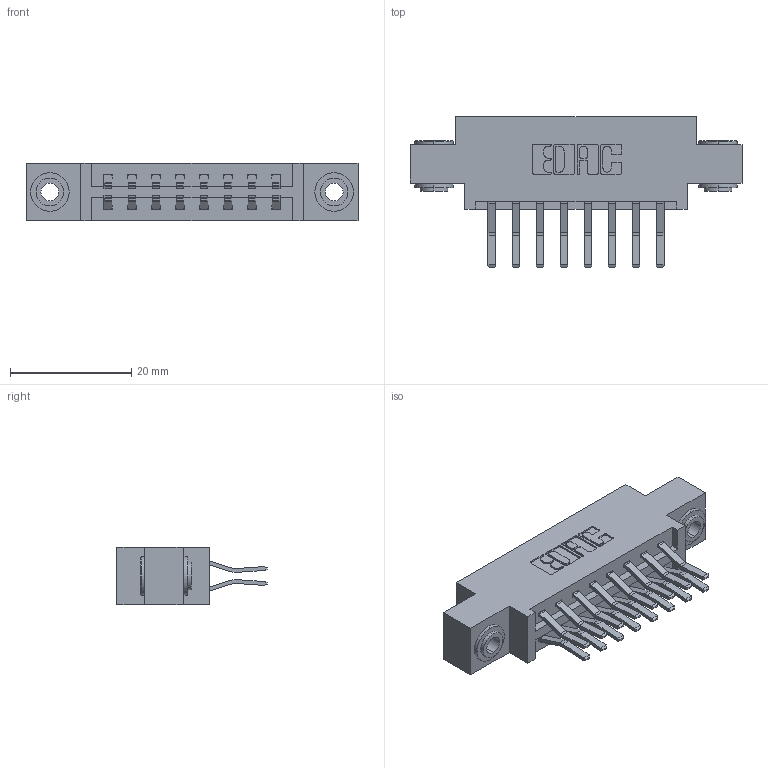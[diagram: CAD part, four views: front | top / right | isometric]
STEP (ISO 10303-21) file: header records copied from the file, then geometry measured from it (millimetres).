
FILE_DESCRIPTION (( 'STEP AP203' ), '1' );
FILE_NAME ('337-016-560-803.STEP', '2019-10-10T18:24:27', ( '' ), ( '' ), 'SwSTEP 2.0', 'SolidWorks 2016', '' );
FILE_SCHEMA (( 'CONFIG_CONTROL_DESIGN' ));
Length unit declared in the file: inch
Products named in the file (4): 345-250-002_345-250-002-102; 345-292-001_560 Tail; 337 Part_0.170 Offset - 0.156 Dia-TH; 337-016-560-803
Assembly tree (19 placements, depth 2):
  337-016-560-803
    337 Part_0.170 Offset - 0.156 Dia-TH
    345-292-001_560 Tail  x16
    345-250-002_345-250-002-102  x2
Bounding box: 54.71 x 24.78 x 9.4 mm (x, y, z)
Volume: 5320.1 mm3; surface area: 6319.9 mm2
Topology: 19 solids, 19 shells, 1052 faces, 3071 edges, 2022 vertices
Faces by surface type: plane 692, cylinder 352, cone 8
Entity records: 11470 total; most frequent: CARTESIAN_POINT 1937, ORIENTED_EDGE 1866, DIRECTION 1747, EDGE_CURVE 933, VECTOR 777, LINE 777, VERTEX_POINT 618, AXIS2_PLACEMENT_3D 485
